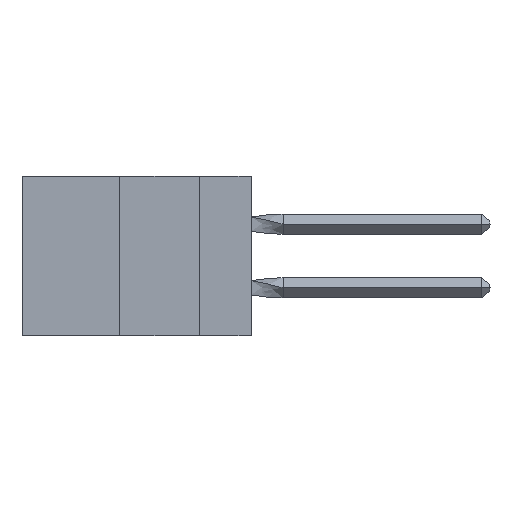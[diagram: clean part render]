
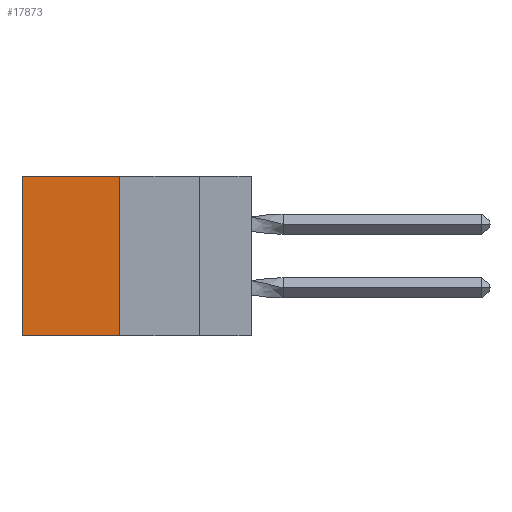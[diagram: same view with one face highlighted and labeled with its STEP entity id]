
A CAD part, left-side view. The second image highlights one B-rep face of the part: STEP entity #17873.
In plain terms, the highlighted planar face has unit normal (-1, 0, 0).
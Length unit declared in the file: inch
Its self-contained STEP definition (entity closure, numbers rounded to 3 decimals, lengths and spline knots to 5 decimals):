
#345 = VERTEX_POINT ( 'NONE', #9972 ) ;
#1178 = LINE ( 'NONE', #14399, #15033 ) ;
#1566 = ORIENTED_EDGE ( 'NONE', *, *, #6012, .F. ) ;
#2734 = VECTOR ( 'NONE', #13052, 39.37008 ) ;
#3169 = EDGE_CURVE ( 'NONE', #7649, #14393, #12147, .T. ) ;
#4079 = AXIS2_PLACEMENT_3D ( 'NONE', #13395, #6099, #6216 ) ;
#4094 = ORIENTED_EDGE ( 'NONE', *, *, #7259, .T. ) ;
#4326 = EDGE_CURVE ( 'NONE', #7649, #6264, #1178, .T. ) ;
#5523 = DIRECTION ( 'NONE',  ( 0., 1., 0. ) ) ;
#6012 = EDGE_CURVE ( 'NONE', #14393, #345, #17869, .T. ) ;
#6099 = DIRECTION ( 'NONE',  ( 1., 0., 0. ) ) ;
#6216 = DIRECTION ( 'NONE',  ( 0., 0., -1. ) ) ;
#6264 = VERTEX_POINT ( 'NONE', #7774 ) ;
#7259 = EDGE_CURVE ( 'NONE', #6264, #345, #16961, .T. ) ;
#7649 = VERTEX_POINT ( 'NONE', #17438 ) ;
#7676 = VECTOR ( 'NONE', #11081, 39.37008 ) ;
#7774 = CARTESIAN_POINT ( 'NONE',  ( 0.305, 0.72, 0. ) ) ;
#8544 = CARTESIAN_POINT ( 'NONE',  ( 0.305, 0.413, -0.5 ) ) ;
#9561 = CARTESIAN_POINT ( 'NONE',  ( 0.305, 0.72, -0.5 ) ) ;
#9972 = CARTESIAN_POINT ( 'NONE',  ( 0.305, 0.72, -0.5 ) ) ;
#10910 = ORIENTED_EDGE ( 'NONE', *, *, #4326, .T. ) ;
#11081 = DIRECTION ( 'NONE',  ( 0., 0., -1. ) ) ;
#11417 = DIRECTION ( 'NONE',  ( 0., 0., -1. ) ) ;
#12147 = LINE ( 'NONE', #8544, #15065 ) ;
#12532 = CARTESIAN_POINT ( 'NONE',  ( 0.305, 0.413, -0.5 ) ) ;
#13052 = DIRECTION ( 'NONE',  ( 0., 1., 0. ) ) ;
#13338 = EDGE_LOOP ( 'NONE', ( #4094, #1566, #17181, #10910 ) ) ;
#13395 = CARTESIAN_POINT ( 'NONE',  ( 0.305, 0.413, -0.5 ) ) ;
#14393 = VERTEX_POINT ( 'NONE', #12532 ) ;
#14399 = CARTESIAN_POINT ( 'NONE',  ( 0.305, 0.413, 0. ) ) ;
#14450 = CARTESIAN_POINT ( 'NONE',  ( 0.305, 0.413, -0.5 ) ) ;
#15033 = VECTOR ( 'NONE', #5523, 39.37008 ) ;
#15065 = VECTOR ( 'NONE', #11417, 39.37008 ) ;
#15373 = FACE_OUTER_BOUND ( 'NONE', #13338, .T. ) ;
#16961 = LINE ( 'NONE', #9561, #7676 ) ;
#17181 = ORIENTED_EDGE ( 'NONE', *, *, #3169, .F. ) ;
#17438 = CARTESIAN_POINT ( 'NONE',  ( 0.305, 0.413, 0. ) ) ;
#17786 = PLANE ( 'NONE',  #4079 ) ;
#17869 = LINE ( 'NONE', #14450, #2734 ) ;
#17873 = ADVANCED_FACE ( 'NONE', ( #15373 ), #17786, .F. ) ;
